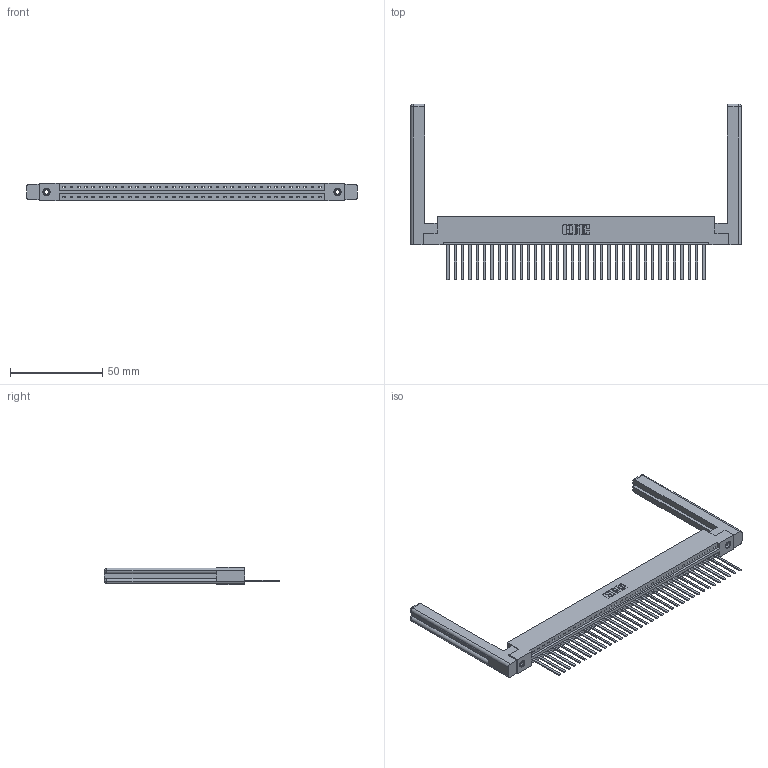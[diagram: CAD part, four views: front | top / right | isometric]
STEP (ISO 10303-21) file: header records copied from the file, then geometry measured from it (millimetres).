
FILE_DESCRIPTION (( 'STEP AP203' ), '1' );
FILE_NAME ('387-036-544-158.STEP', '2019-10-04T13:47:43', ( '' ), ( '' ), 'SwSTEP 2.0', 'SolidWorks 2016', '' );
FILE_SCHEMA (( 'CONFIG_CONTROL_DESIGN' ));
Length unit declared in the file: inch
Products named in the file (5): 345-292-001_345-293-144; 307-220-058; 387-036-544-158; 345-250-001_345-250-001-102; 337 Part_Flush Mounting Lugs - 0.156 Dia-TI
Assembly tree (41 placements, depth 2):
  387-036-544-158
    337 Part_Flush Mounting Lugs - 0.156 Dia-TI
    345-292-001_345-293-144  x36
    345-250-001_345-250-001-102  x2
    307-220-058  x2
Bounding box: 179.27 x 95.38 x 9.4 mm (x, y, z)
Volume: 26136.4 mm3; surface area: 26158.4 mm2
Topology: 41 solids, 41 shells, 2272 faces, 6785 edges, 4462 vertices
Faces by surface type: plane 1666, cylinder 582, cone 12, torus 12
Entity records: 29986 total; most frequent: CARTESIAN_POINT 5221, ORIENTED_EDGE 5132, DIRECTION 4422, EDGE_CURVE 2566, VECTOR 2394, LINE 2394, VERTEX_POINT 1702, AXIS2_PLACEMENT_3D 1014
